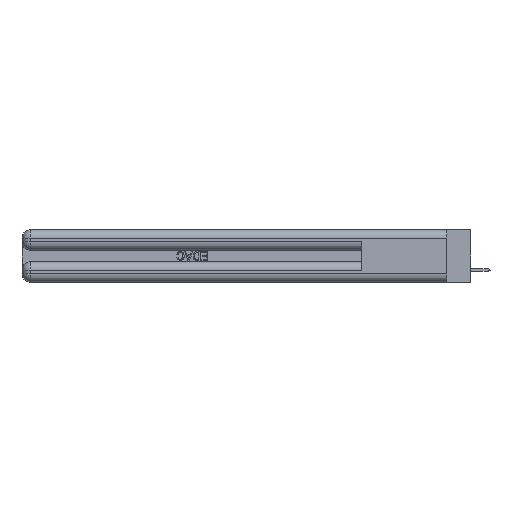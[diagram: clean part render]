
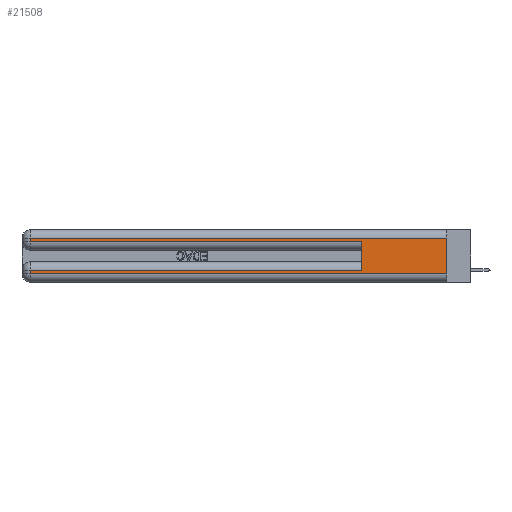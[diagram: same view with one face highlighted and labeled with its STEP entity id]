
A CAD part, left-side view. The second image highlights one B-rep face of the part: STEP entity #21508.
In plain terms, the highlighted planar face has unit normal (-1, 0, 0).
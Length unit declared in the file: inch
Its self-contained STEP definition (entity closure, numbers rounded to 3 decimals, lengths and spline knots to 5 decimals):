
#412 = LINE ( 'NONE', #35265, #35948 ) ;
#538 = FACE_OUTER_BOUND ( 'NONE', #20899, .T. ) ;
#1046 = DIRECTION ( 'NONE',  ( 0., 0., 1. ) ) ;
#1311 = VECTOR ( 'NONE', #34814, 39.37008 ) ;
#2801 = LINE ( 'NONE', #34630, #1311 ) ;
#3903 = CARTESIAN_POINT ( 'NONE',  ( 0., 2.94, 0.31 ) ) ;
#4549 = VERTEX_POINT ( 'NONE', #3903 ) ;
#5266 = EDGE_CURVE ( 'NONE', #31800, #4549, #18807, .T. ) ;
#5365 = DIRECTION ( 'NONE',  ( 0., 0., -1. ) ) ;
#5681 = PLANE ( 'NONE',  #16260 ) ;
#7404 = EDGE_CURVE ( 'NONE', #11302, #33704, #8985, .T. ) ;
#8985 = LINE ( 'NONE', #11835, #10738 ) ;
#10490 = VECTOR ( 'NONE', #34551, 39.37008 ) ;
#10738 = VECTOR ( 'NONE', #15455, 39.37008 ) ;
#11253 = LINE ( 'NONE', #36984, #30312 ) ;
#11302 = VERTEX_POINT ( 'NONE', #31829 ) ;
#11835 = CARTESIAN_POINT ( 'NONE',  ( 0., 0., 0.085 ) ) ;
#12031 = CARTESIAN_POINT ( 'NONE',  ( 0., 0., 0.285 ) ) ;
#12037 = VECTOR ( 'NONE', #1046, 39.37008 ) ;
#12275 = CARTESIAN_POINT ( 'NONE',  ( 0., 2.94, 0.06 ) ) ;
#12989 = CARTESIAN_POINT ( 'NONE',  ( 0., 2.94, 0.085 ) ) ;
#13119 = CARTESIAN_POINT ( 'NONE',  ( 0., 2.94, 0.285 ) ) ;
#14368 = EDGE_CURVE ( 'NONE', #4549, #14390, #24370, .T. ) ;
#14390 = VERTEX_POINT ( 'NONE', #13119 ) ;
#14652 = EDGE_CURVE ( 'NONE', #23420, #21847, #2801, .T. ) ;
#15455 = DIRECTION ( 'NONE',  ( 0., 1., 0. ) ) ;
#15743 = DIRECTION ( 'NONE',  ( 0., 1., 0. ) ) ;
#15762 = ORIENTED_EDGE ( 'NONE', *, *, #24105, .T. ) ;
#16260 = AXIS2_PLACEMENT_3D ( 'NONE', #26446, #17865, #31983 ) ;
#17206 = LINE ( 'NONE', #12031, #10490 ) ;
#17865 = DIRECTION ( 'NONE',  ( 1., 0., 0. ) ) ;
#18807 = LINE ( 'NONE', #33102, #35258 ) ;
#20421 = ORIENTED_EDGE ( 'NONE', *, *, #7404, .T. ) ;
#20899 = EDGE_LOOP ( 'NONE', ( #35370, #34164, #36060, #35827, #33634, #20421, #15762, #34115 ) ) ;
#20979 = DIRECTION ( 'NONE',  ( 0., 0., -1. ) ) ;
#21508 = ADVANCED_FACE ( 'NONE', ( #538 ), #5681, .F. ) ;
#21847 = VERTEX_POINT ( 'NONE', #31004 ) ;
#22219 = EDGE_CURVE ( 'NONE', #11302, #23034, #30017, .T. ) ;
#23034 = VERTEX_POINT ( 'NONE', #24150 ) ;
#23420 = VERTEX_POINT ( 'NONE', #12275 ) ;
#24105 = EDGE_CURVE ( 'NONE', #33704, #23420, #11253, .T. ) ;
#24150 = CARTESIAN_POINT ( 'NONE',  ( 0., 0.6, 0.285 ) ) ;
#24370 = LINE ( 'NONE', #25132, #24413 ) ;
#24413 = VECTOR ( 'NONE', #36746, 39.37008 ) ;
#25132 = CARTESIAN_POINT ( 'NONE',  ( 0., 2.94, 0.37 ) ) ;
#26446 = CARTESIAN_POINT ( 'NONE',  ( 0., 0., 0.37 ) ) ;
#27137 = EDGE_CURVE ( 'NONE', #31800, #21847, #412, .T. ) ;
#27155 = CARTESIAN_POINT ( 'NONE',  ( 0., 0.6, 0.145 ) ) ;
#30017 = LINE ( 'NONE', #27155, #12037 ) ;
#30312 = VECTOR ( 'NONE', #5365, 39.37008 ) ;
#30786 = EDGE_CURVE ( 'NONE', #14390, #23034, #17206, .T. ) ;
#31004 = CARTESIAN_POINT ( 'NONE',  ( 0., 0., 0.06 ) ) ;
#31800 = VERTEX_POINT ( 'NONE', #33855 ) ;
#31829 = CARTESIAN_POINT ( 'NONE',  ( 0., 0.6, 0.085 ) ) ;
#31983 = DIRECTION ( 'NONE',  ( 0., 0., -1. ) ) ;
#33102 = CARTESIAN_POINT ( 'NONE',  ( 0., 0., 0.31 ) ) ;
#33634 = ORIENTED_EDGE ( 'NONE', *, *, #22219, .F. ) ;
#33704 = VERTEX_POINT ( 'NONE', #12989 ) ;
#33855 = CARTESIAN_POINT ( 'NONE',  ( 0., 0., 0.31 ) ) ;
#34115 = ORIENTED_EDGE ( 'NONE', *, *, #14652, .T. ) ;
#34164 = ORIENTED_EDGE ( 'NONE', *, *, #5266, .T. ) ;
#34551 = DIRECTION ( 'NONE',  ( 0., -1., 0. ) ) ;
#34630 = CARTESIAN_POINT ( 'NONE',  ( 0., 0., 0.06 ) ) ;
#34814 = DIRECTION ( 'NONE',  ( 0., -1., 0. ) ) ;
#35258 = VECTOR ( 'NONE', #15743, 39.37008 ) ;
#35265 = CARTESIAN_POINT ( 'NONE',  ( 0., 0., 0.37 ) ) ;
#35370 = ORIENTED_EDGE ( 'NONE', *, *, #27137, .F. ) ;
#35827 = ORIENTED_EDGE ( 'NONE', *, *, #30786, .T. ) ;
#35948 = VECTOR ( 'NONE', #20979, 39.37008 ) ;
#36060 = ORIENTED_EDGE ( 'NONE', *, *, #14368, .T. ) ;
#36746 = DIRECTION ( 'NONE',  ( 0., 0., -1. ) ) ;
#36984 = CARTESIAN_POINT ( 'NONE',  ( 0., 2.94, 0.37 ) ) ;
